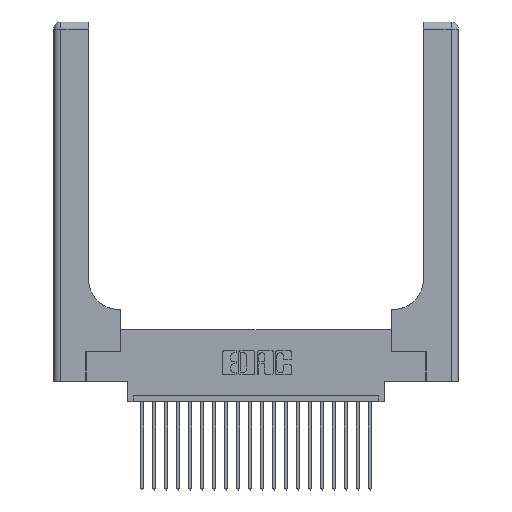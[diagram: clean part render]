
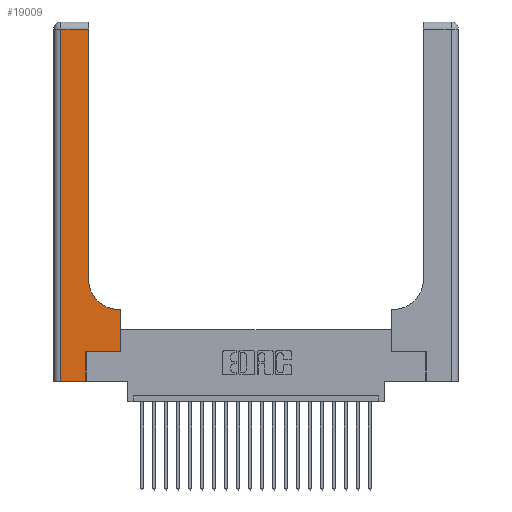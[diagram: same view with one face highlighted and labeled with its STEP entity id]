
A CAD part, top view. The second image highlights one B-rep face of the part: STEP entity #19009.
In plain terms, the highlighted planar face has unit normal (0, 0, 1).
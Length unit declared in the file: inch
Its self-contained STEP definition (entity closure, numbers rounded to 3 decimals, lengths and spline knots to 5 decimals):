
#63 = EDGE_CURVE ( 'NONE', #19566, #4627, #4295, .T. ) ;
#222 = EDGE_CURVE ( 'NONE', #5109, #15387, #5961, .T. ) ;
#280 = LINE ( 'NONE', #11475, #16397 ) ;
#674 = DIRECTION ( 'NONE',  ( 0., 1., 0. ) ) ;
#798 = EDGE_CURVE ( 'NONE', #4627, #21856, #4778, .T. ) ;
#1180 = ORIENTED_EDGE ( 'NONE', *, *, #798, .T. ) ;
#1732 = CARTESIAN_POINT ( 'NONE',  ( 0.06, 3., 0.37 ) ) ;
#1936 = VERTEX_POINT ( 'NONE', #4415 ) ;
#2134 = ORIENTED_EDGE ( 'NONE', *, *, #9066, .T. ) ;
#2709 = DIRECTION ( 'NONE',  ( -1., 0., 0. ) ) ;
#3147 = VECTOR ( 'NONE', #12999, 39.37008 ) ;
#3270 = VECTOR ( 'NONE', #5446, 39.37008 ) ;
#3598 = EDGE_CURVE ( 'NONE', #14255, #1936, #10845, .T. ) ;
#3879 = ORIENTED_EDGE ( 'NONE', *, *, #63, .T. ) ;
#4117 = CARTESIAN_POINT ( 'NONE',  ( 0.2915, 0.6, 0.37 ) ) ;
#4172 = DIRECTION ( 'NONE',  ( 1., 0., 0. ) ) ;
#4295 = LINE ( 'NONE', #4117, #3147 ) ;
#4415 = CARTESIAN_POINT ( 'NONE',  ( 0.06, 2.94, 0.37 ) ) ;
#4627 = VERTEX_POINT ( 'NONE', #6763 ) ;
#4686 = VECTOR ( 'NONE', #4172, 39.37008 ) ;
#4778 = CIRCLE ( 'NONE', #10228, 0.25 ) ;
#5109 = VERTEX_POINT ( 'NONE', #9665 ) ;
#5446 = DIRECTION ( 'NONE',  ( 0., -1., 0. ) ) ;
#5961 = LINE ( 'NONE', #6919, #22322 ) ;
#6129 = ORIENTED_EDGE ( 'NONE', *, *, #17162, .T. ) ;
#6743 = DIRECTION ( 'NONE',  ( -1., 0., 0. ) ) ;
#6763 = CARTESIAN_POINT ( 'NONE',  ( 0.5415, 0.6, 0.37 ) ) ;
#6766 = EDGE_CURVE ( 'NONE', #15387, #18382, #280, .T. ) ;
#6919 = CARTESIAN_POINT ( 'NONE',  ( 0., 0., 0.37 ) ) ;
#6938 = AXIS2_PLACEMENT_3D ( 'NONE', #17736, #23131, #6743 ) ;
#7003 = EDGE_LOOP ( 'NONE', ( #6129, #15332, #19064, #14195, #18576, #2134, #16076, #3879, #1180 ) ) ;
#8083 = CARTESIAN_POINT ( 'NONE',  ( 0.2915, 3., 0.37 ) ) ;
#9066 = EDGE_CURVE ( 'NONE', #18382, #18533, #11723, .T. ) ;
#9268 = CARTESIAN_POINT ( 'NONE',  ( 0.5585, 0.25, 0.37 ) ) ;
#9665 = CARTESIAN_POINT ( 'NONE',  ( 0.06, 0., 0.37 ) ) ;
#10073 = EDGE_CURVE ( 'NONE', #1936, #5109, #13411, .T. ) ;
#10228 = AXIS2_PLACEMENT_3D ( 'NONE', #17443, #13751, #11786 ) ;
#10581 = CARTESIAN_POINT ( 'NONE',  ( 0.2915, 0.85, 0.37 ) ) ;
#10704 = LINE ( 'NONE', #9268, #13791 ) ;
#10845 = LINE ( 'NONE', #20716, #15934 ) ;
#11475 = CARTESIAN_POINT ( 'NONE',  ( 0.269, 0., 0.37 ) ) ;
#11560 = DIRECTION ( 'NONE',  ( 0., 1., 0. ) ) ;
#11723 = LINE ( 'NONE', #22136, #4686 ) ;
#11786 = DIRECTION ( 'NONE',  ( 1., 0., 0. ) ) ;
#12999 = DIRECTION ( 'NONE',  ( -1., 0., 0. ) ) ;
#13411 = LINE ( 'NONE', #1732, #3270 ) ;
#13751 = DIRECTION ( 'NONE',  ( 0., 0., -1. ) ) ;
#13791 = VECTOR ( 'NONE', #21909, 39.37008 ) ;
#14195 = ORIENTED_EDGE ( 'NONE', *, *, #222, .T. ) ;
#14255 = VERTEX_POINT ( 'NONE', #16942 ) ;
#15332 = ORIENTED_EDGE ( 'NONE', *, *, #3598, .T. ) ;
#15387 = VERTEX_POINT ( 'NONE', #19238 ) ;
#15605 = PLANE ( 'NONE',  #6938 ) ;
#15924 = DIRECTION ( 'NONE',  ( 1., 0., 0. ) ) ;
#15934 = VECTOR ( 'NONE', #2709, 39.37008 ) ;
#16076 = ORIENTED_EDGE ( 'NONE', *, *, #16319, .T. ) ;
#16319 = EDGE_CURVE ( 'NONE', #18533, #19566, #10704, .T. ) ;
#16397 = VECTOR ( 'NONE', #11560, 39.37008 ) ;
#16626 = FACE_OUTER_BOUND ( 'NONE', #7003, .T. ) ;
#16942 = CARTESIAN_POINT ( 'NONE',  ( 0.2915, 2.94, 0.37 ) ) ;
#17162 = EDGE_CURVE ( 'NONE', #21856, #14255, #21250, .T. ) ;
#17443 = CARTESIAN_POINT ( 'NONE',  ( 0.5415, 0.85, 0.37 ) ) ;
#17736 = CARTESIAN_POINT ( 'NONE',  ( 0., 3., 0.37 ) ) ;
#18382 = VERTEX_POINT ( 'NONE', #21456 ) ;
#18455 = CARTESIAN_POINT ( 'NONE',  ( 0.5585, 0.6, 0.37 ) ) ;
#18533 = VERTEX_POINT ( 'NONE', #21840 ) ;
#18576 = ORIENTED_EDGE ( 'NONE', *, *, #6766, .T. ) ;
#19009 = ADVANCED_FACE ( 'NONE', ( #16626 ), #15605, .F. ) ;
#19064 = ORIENTED_EDGE ( 'NONE', *, *, #10073, .T. ) ;
#19238 = CARTESIAN_POINT ( 'NONE',  ( 0.269, 0., 0.37 ) ) ;
#19566 = VERTEX_POINT ( 'NONE', #18455 ) ;
#20716 = CARTESIAN_POINT ( 'NONE',  ( 0., 2.94, 0.37 ) ) ;
#21250 = LINE ( 'NONE', #8083, #21813 ) ;
#21456 = CARTESIAN_POINT ( 'NONE',  ( 0.269, 0.25, 0.37 ) ) ;
#21813 = VECTOR ( 'NONE', #674, 39.37008 ) ;
#21840 = CARTESIAN_POINT ( 'NONE',  ( 0.5585, 0.25, 0.37 ) ) ;
#21856 = VERTEX_POINT ( 'NONE', #10581 ) ;
#21909 = DIRECTION ( 'NONE',  ( 0., 1., 0. ) ) ;
#22136 = CARTESIAN_POINT ( 'NONE',  ( 0.269, 0.25, 0.37 ) ) ;
#22322 = VECTOR ( 'NONE', #15924, 39.37008 ) ;
#23131 = DIRECTION ( 'NONE',  ( 0., 0., -1. ) ) ;
